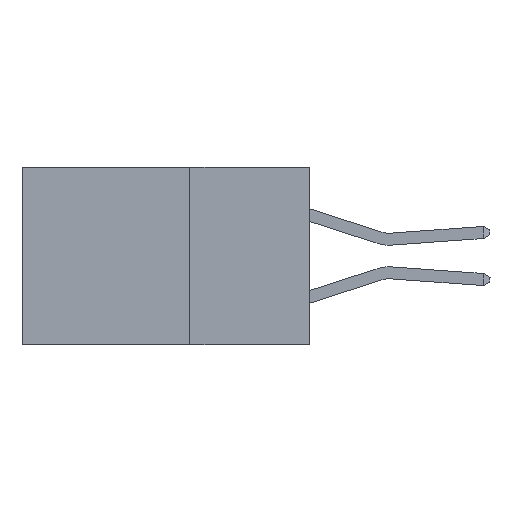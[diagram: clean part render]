
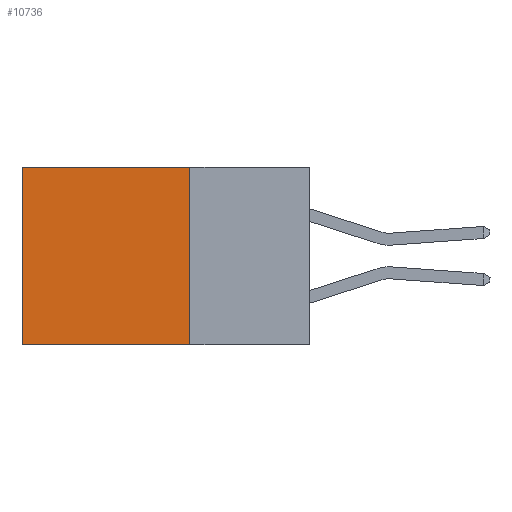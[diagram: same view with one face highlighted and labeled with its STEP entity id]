
A CAD part, left-side view. The second image highlights one B-rep face of the part: STEP entity #10736.
In plain terms, the highlighted planar face has unit normal (-1, 0, 0).
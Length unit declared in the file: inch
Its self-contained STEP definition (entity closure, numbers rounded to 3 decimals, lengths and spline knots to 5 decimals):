
#107 = VERTEX_POINT ( 'NONE', #9429 ) ;
#202 = VECTOR ( 'NONE', #2613, 39.37008 ) ;
#575 = DIRECTION ( 'NONE',  ( 0., 0., -1. ) ) ;
#1193 = EDGE_CURVE ( 'NONE', #10400, #10179, #2743, .T. ) ;
#2221 = LINE ( 'NONE', #2568, #202 ) ;
#2522 = DIRECTION ( 'NONE',  ( 0., 0., -1. ) ) ;
#2568 = CARTESIAN_POINT ( 'NONE',  ( 0.298, 0.25, 0. ) ) ;
#2613 = DIRECTION ( 'NONE',  ( 0., 1., 0. ) ) ;
#2743 = LINE ( 'NONE', #9046, #13758 ) ;
#3025 = CARTESIAN_POINT ( 'NONE',  ( 0.298, 0.25, -0.37 ) ) ;
#3097 = EDGE_CURVE ( 'NONE', #107, #10400, #2221, .T. ) ;
#3592 = EDGE_CURVE ( 'NONE', #11553, #10179, #12375, .T. ) ;
#3723 = FACE_OUTER_BOUND ( 'NONE', #13697, .T. ) ;
#4572 = CARTESIAN_POINT ( 'NONE',  ( 0.298, 0.25, 0. ) ) ;
#5036 = LINE ( 'NONE', #5547, #6551 ) ;
#5547 = CARTESIAN_POINT ( 'NONE',  ( 0.298, 0.25, 0. ) ) ;
#6067 = CARTESIAN_POINT ( 'NONE',  ( 0.298, 0.25, -0.37 ) ) ;
#6551 = VECTOR ( 'NONE', #6687, 39.37008 ) ;
#6687 = DIRECTION ( 'NONE',  ( 0., 0., -1. ) ) ;
#6708 = CARTESIAN_POINT ( 'NONE',  ( 0.298, 0.6, 0. ) ) ;
#6801 = ORIENTED_EDGE ( 'NONE', *, *, #12369, .F. ) ;
#6994 = PLANE ( 'NONE',  #8431 ) ;
#7563 = ORIENTED_EDGE ( 'NONE', *, *, #3592, .F. ) ;
#8431 = AXIS2_PLACEMENT_3D ( 'NONE', #4572, #13101, #575 ) ;
#8587 = CARTESIAN_POINT ( 'NONE',  ( 0.298, 0.6, -0.37 ) ) ;
#9046 = CARTESIAN_POINT ( 'NONE',  ( 0.298, 0.6, 0. ) ) ;
#9305 = ORIENTED_EDGE ( 'NONE', *, *, #1193, .T. ) ;
#9429 = CARTESIAN_POINT ( 'NONE',  ( 0.298, 0.25, 0. ) ) ;
#9574 = VECTOR ( 'NONE', #10654, 39.37008 ) ;
#10179 = VERTEX_POINT ( 'NONE', #8587 ) ;
#10400 = VERTEX_POINT ( 'NONE', #6708 ) ;
#10654 = DIRECTION ( 'NONE',  ( 0., 1., 0. ) ) ;
#10736 = ADVANCED_FACE ( 'NONE', ( #3723 ), #6994, .F. ) ;
#11553 = VERTEX_POINT ( 'NONE', #6067 ) ;
#12369 = EDGE_CURVE ( 'NONE', #107, #11553, #5036, .T. ) ;
#12375 = LINE ( 'NONE', #3025, #9574 ) ;
#12521 = ORIENTED_EDGE ( 'NONE', *, *, #3097, .T. ) ;
#13101 = DIRECTION ( 'NONE',  ( 1., 0., 0. ) ) ;
#13697 = EDGE_LOOP ( 'NONE', ( #9305, #7563, #6801, #12521 ) ) ;
#13758 = VECTOR ( 'NONE', #2522, 39.37008 ) ;
